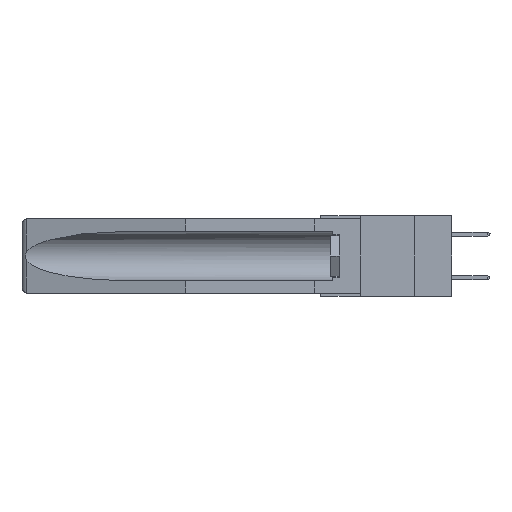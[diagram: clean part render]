
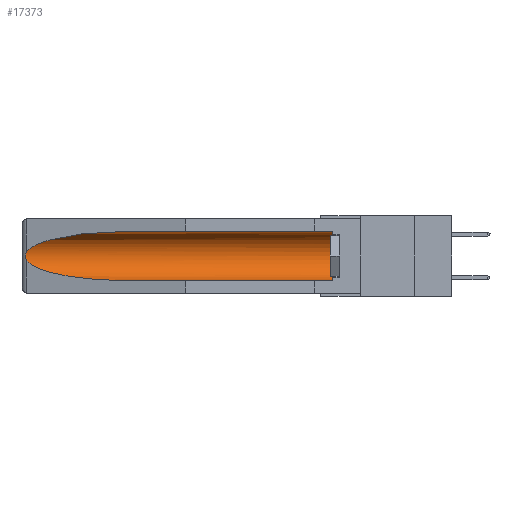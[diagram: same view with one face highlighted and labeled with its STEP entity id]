
A CAD part, left-side view. The second image highlights one B-rep face of the part: STEP entity #17373.
In plain terms, the highlighted cylindrical face has radius 2.857 mm (diameter 5.715 mm), a partial arc.
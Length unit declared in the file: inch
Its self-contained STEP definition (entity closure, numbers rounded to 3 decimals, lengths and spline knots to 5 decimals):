
#557 = LINE ( 'NONE', #12955, #6051 ) ;
#595 = CARTESIAN_POINT ( 'NONE',  ( 0.2673, 1.5327, -0.16383 ) ) ;
#729 = VERTEX_POINT ( 'NONE', #4858 ) ;
#1340 = ORIENTED_EDGE ( 'NONE', *, *, #15209, .F. ) ;
#2001 = DIRECTION ( 'NONE',  ( 0., 1., 0. ) ) ;
#2297 = CARTESIAN_POINT ( 'NONE',  ( 0.25451, 1.48313, -0.24835 ) ) ;
#2953 = CARTESIAN_POINT ( 'NONE',  ( 0.25451, 1.48313, -0.09465 ) ) ;
#3598 =( BOUNDED_CURVE ( )  B_SPLINE_CURVE ( 3, ( #15598, #15768, #2953, #19413 ),
 .UNSPECIFIED., .F., .F. ) 
 B_SPLINE_CURVE_WITH_KNOTS ( ( 4, 4 ),
 ( 4.71239, 6.08839 ),
 .UNSPECIFIED. ) 
 CURVE ( )  GEOMETRIC_REPRESENTATION_ITEM ( )  RATIONAL_B_SPLINE_CURVE ( ( 1., 0.848, 0.848, 1. ) ) 
 REPRESENTATION_ITEM ( '' )  );
#3858 = EDGE_CURVE ( 'NONE', #9666, #729, #557, .T. ) ;
#4138 = CARTESIAN_POINT ( 'NONE',  ( 0.2675, 1.53308, -0.17534 ) ) ;
#4458 = DIRECTION ( 'NONE',  ( 0., 1., 0. ) ) ;
#4780 = CARTESIAN_POINT ( 'NONE',  ( 0.155, 0.126, -0.1715 ) ) ;
#4787 = CARTESIAN_POINT ( 'NONE',  ( 0.26537, 1.52718, -0.14972 ) ) ;
#4858 = CARTESIAN_POINT ( 'NONE',  ( 0.155, 1.07973, -0.059 ) ) ;
#5587 = EDGE_LOOP ( 'NONE', ( #16489, #13392, #16420, #1340, #18296, #7771 ) ) ;
#5833 = CARTESIAN_POINT ( 'NONE',  ( 0.26537, 1.52718, -0.19328 ) ) ;
#6051 = VECTOR ( 'NONE', #13191, 39.37008 ) ;
#6318 = CARTESIAN_POINT ( 'NONE',  ( 0.26537, 1.52718, -0.14972 ) ) ;
#6418 = CYLINDRICAL_SURFACE ( 'NONE', #14954, 0.1125 ) ;
#6432 = VERTEX_POINT ( 'NONE', #14566 ) ;
#7771 = ORIENTED_EDGE ( 'NONE', *, *, #3858, .T. ) ;
#7825 = CARTESIAN_POINT ( 'NONE',  ( 0.2675, 1.53308, -0.16763 ) ) ;
#8758 = EDGE_CURVE ( 'NONE', #6432, #9666, #15503, .T. ) ;
#8794 = VECTOR ( 'NONE', #4458, 39.37008 ) ;
#9666 = VERTEX_POINT ( 'NONE', #11391 ) ;
#9940 = CARTESIAN_POINT ( 'NONE',  ( 0.155, 1.07973, -0.284 ) ) ;
#10078 = DIRECTION ( 'NONE',  ( 0., 0., 1. ) ) ;
#10205 = CARTESIAN_POINT ( 'NONE',  ( 0.26537, 1.52718, -0.19328 ) ) ;
#10355 = FACE_OUTER_BOUND ( 'NONE', #5587, .T. ) ;
#11144 = CARTESIAN_POINT ( 'NONE',  ( 0.155, 1.07973, -0.284 ) ) ;
#11391 = CARTESIAN_POINT ( 'NONE',  ( 0.155, 0.126, -0.059 ) ) ;
#11463 = CARTESIAN_POINT ( 'NONE',  ( 0.26537, 1.52718, -0.19328 ) ) ;
#12362 = B_SPLINE_CURVE_WITH_KNOTS ( 'NONE', 3,
 ( #6318, #19067, #15075, #595, #7825, #4138, #16894, #18747, #20574, #11463 ),
 .UNSPECIFIED., .F., .F.,
 ( 4, 2, 2, 2, 4 ),
 ( 0., 0.00029, 0.00058, 0.00087, 0.00117 ),
 .UNSPECIFIED. ) ;
#12553 = VERTEX_POINT ( 'NONE', #9940 ) ;
#12955 = CARTESIAN_POINT ( 'NONE',  ( 0.155, -0.30754, -0.059 ) ) ;
#13139 = CARTESIAN_POINT ( 'NONE',  ( 0.21114, 1.30732, -0.284 ) ) ;
#13191 = DIRECTION ( 'NONE',  ( 0., 1., 0. ) ) ;
#13392 = ORIENTED_EDGE ( 'NONE', *, *, #18100, .T. ) ;
#13605 = AXIS2_PLACEMENT_3D ( 'NONE', #4780, #21308, #10078 ) ;
#14513 = VERTEX_POINT ( 'NONE', #10205 ) ;
#14566 = CARTESIAN_POINT ( 'NONE',  ( 0.155, 0.126, -0.284 ) ) ;
#14954 = AXIS2_PLACEMENT_3D ( 'NONE', #19953, #2001, #16513 ) ;
#15075 = CARTESIAN_POINT ( 'NONE',  ( 0.26654, 1.53092, -0.15636 ) ) ;
#15209 = EDGE_CURVE ( 'NONE', #6432, #12553, #21583, .T. ) ;
#15296 = CARTESIAN_POINT ( 'NONE',  ( 0.155, -0.30754, -0.284 ) ) ;
#15503 = CIRCLE ( 'NONE', #13605, 0.1125 ) ;
#15598 = CARTESIAN_POINT ( 'NONE',  ( 0.155, 1.07973, -0.059 ) ) ;
#15768 = CARTESIAN_POINT ( 'NONE',  ( 0.21114, 1.30732, -0.059 ) ) ;
#16420 = ORIENTED_EDGE ( 'NONE', *, *, #18596, .T. ) ;
#16489 = ORIENTED_EDGE ( 'NONE', *, *, #21579, .T. ) ;
#16513 = DIRECTION ( 'NONE',  ( 0., 0., 1. ) ) ;
#16894 = CARTESIAN_POINT ( 'NONE',  ( 0.2673, 1.53269, -0.17917 ) ) ;
#17373 = ADVANCED_FACE ( 'NONE', ( #10355 ), #6418, .F. ) ;
#18100 = EDGE_CURVE ( 'NONE', #18732, #14513, #12362, .T. ) ;
#18296 = ORIENTED_EDGE ( 'NONE', *, *, #8758, .T. ) ;
#18596 = EDGE_CURVE ( 'NONE', #14513, #12553, #20569, .T. ) ;
#18732 = VERTEX_POINT ( 'NONE', #4787 ) ;
#18747 = CARTESIAN_POINT ( 'NONE',  ( 0.26655, 1.53094, -0.18657 ) ) ;
#19067 = CARTESIAN_POINT ( 'NONE',  ( 0.26597, 1.52961, -0.15275 ) ) ;
#19413 = CARTESIAN_POINT ( 'NONE',  ( 0.26537, 1.52718, -0.14972 ) ) ;
#19953 = CARTESIAN_POINT ( 'NONE',  ( 0.155, -0.30754, -0.1715 ) ) ;
#20569 =( BOUNDED_CURVE ( )  B_SPLINE_CURVE ( 3, ( #5833, #2297, #13139, #11144 ),
 .UNSPECIFIED., .F., .F. ) 
 B_SPLINE_CURVE_WITH_KNOTS ( ( 4, 4 ),
 ( 0.1948, 1.5708 ),
 .UNSPECIFIED. ) 
 CURVE ( )  GEOMETRIC_REPRESENTATION_ITEM ( )  RATIONAL_B_SPLINE_CURVE ( ( 1., 0.848, 0.848, 1. ) ) 
 REPRESENTATION_ITEM ( '' )  );
#20574 = CARTESIAN_POINT ( 'NONE',  ( 0.26597, 1.5296, -0.19026 ) ) ;
#21308 = DIRECTION ( 'NONE',  ( 0., -1., 0. ) ) ;
#21579 = EDGE_CURVE ( 'NONE', #729, #18732, #3598, .T. ) ;
#21583 = LINE ( 'NONE', #15296, #8794 ) ;
